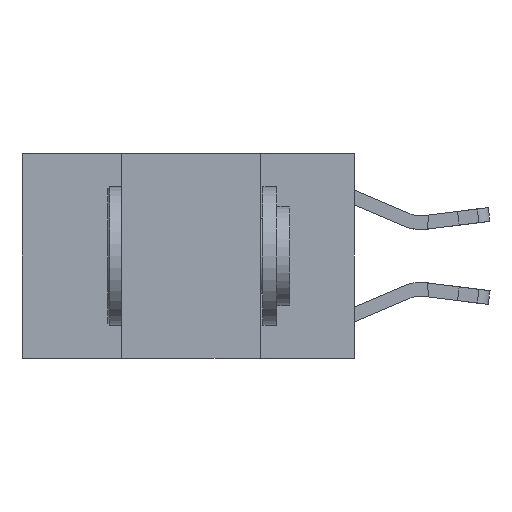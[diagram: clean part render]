
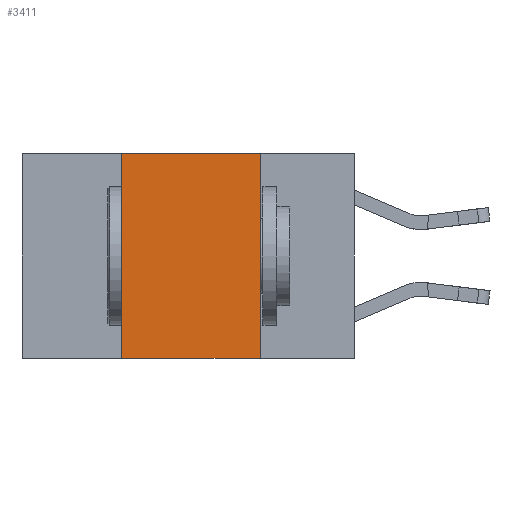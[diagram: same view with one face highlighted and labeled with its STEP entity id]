
A CAD part, left-side view. The second image highlights one B-rep face of the part: STEP entity #3411.
In plain terms, the highlighted planar face has unit normal (-1, 0, 0).
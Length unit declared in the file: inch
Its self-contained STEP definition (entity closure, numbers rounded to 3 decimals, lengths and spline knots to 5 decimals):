
#657 = VERTEX_POINT ( 'NONE', #14729 ) ;
#900 = DIRECTION ( 'NONE',  ( 0., -1., 0. ) ) ;
#1626 = VECTOR ( 'NONE', #14368, 39.37008 ) ;
#2555 = DIRECTION ( 'NONE',  ( 1., 0., 0. ) ) ;
#3411 = ADVANCED_FACE ( 'NONE', ( #17100 ), #15183, .F. ) ;
#3640 = EDGE_LOOP ( 'NONE', ( #7985, #19699, #3686, #9302 ) ) ;
#3686 = ORIENTED_EDGE ( 'NONE', *, *, #25296, .F. ) ;
#3836 = EDGE_CURVE ( 'NONE', #15007, #15060, #12192, .T. ) ;
#5166 = CARTESIAN_POINT ( 'NONE',  ( 0., 0.6, 0. ) ) ;
#5542 = AXIS2_PLACEMENT_3D ( 'NONE', #23361, #2555, #17247 ) ;
#7138 = CARTESIAN_POINT ( 'NONE',  ( 0., 0.17, 0. ) ) ;
#7985 = ORIENTED_EDGE ( 'NONE', *, *, #3836, .F. ) ;
#9302 = ORIENTED_EDGE ( 'NONE', *, *, #17013, .T. ) ;
#9455 = CARTESIAN_POINT ( 'NONE',  ( 0., 0.17, -0.37 ) ) ;
#12192 = LINE ( 'NONE', #26673, #1626 ) ;
#12470 = CARTESIAN_POINT ( 'NONE',  ( 0., 0.42, 0. ) ) ;
#13065 = EDGE_CURVE ( 'NONE', #17201, #15007, #19026, .T. ) ;
#13518 = VECTOR ( 'NONE', #900, 39.37008 ) ;
#13880 = CARTESIAN_POINT ( 'NONE',  ( 0., 0.6, -0.37 ) ) ;
#14025 = VECTOR ( 'NONE', #24148, 39.37008 ) ;
#14108 = LINE ( 'NONE', #23581, #24413 ) ;
#14368 = DIRECTION ( 'NONE',  ( 0., 0., -1. ) ) ;
#14729 = CARTESIAN_POINT ( 'NONE',  ( 0., 0.42, -0.37 ) ) ;
#15007 = VERTEX_POINT ( 'NONE', #7138 ) ;
#15060 = VERTEX_POINT ( 'NONE', #9455 ) ;
#15183 = PLANE ( 'NONE',  #5542 ) ;
#17013 = EDGE_CURVE ( 'NONE', #657, #15060, #20153, .T. ) ;
#17100 = FACE_OUTER_BOUND ( 'NONE', #3640, .T. ) ;
#17201 = VERTEX_POINT ( 'NONE', #12470 ) ;
#17247 = DIRECTION ( 'NONE',  ( 0., 0., -1. ) ) ;
#17377 = DIRECTION ( 'NONE',  ( 0., 0., 1. ) ) ;
#19026 = LINE ( 'NONE', #5166, #13518 ) ;
#19699 = ORIENTED_EDGE ( 'NONE', *, *, #13065, .F. ) ;
#20153 = LINE ( 'NONE', #13880, #14025 ) ;
#23361 = CARTESIAN_POINT ( 'NONE',  ( 0., 0.6, 0. ) ) ;
#23581 = CARTESIAN_POINT ( 'NONE',  ( 0., 0.42, 0. ) ) ;
#24148 = DIRECTION ( 'NONE',  ( 0., -1., 0. ) ) ;
#24413 = VECTOR ( 'NONE', #17377, 39.37008 ) ;
#25296 = EDGE_CURVE ( 'NONE', #657, #17201, #14108, .T. ) ;
#26673 = CARTESIAN_POINT ( 'NONE',  ( 0., 0.17, 0. ) ) ;
